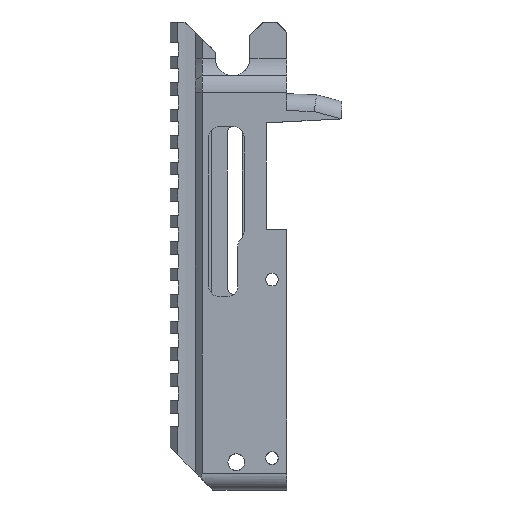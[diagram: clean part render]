
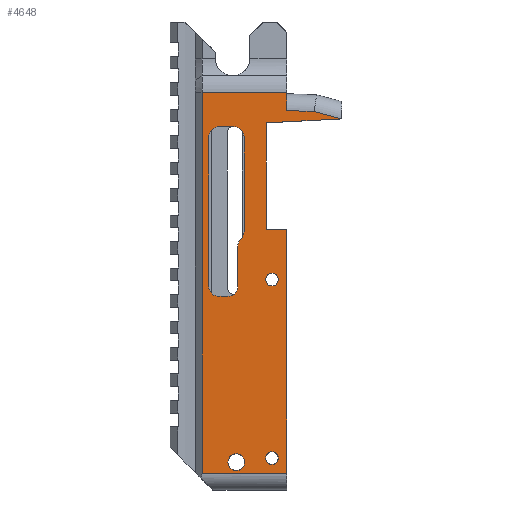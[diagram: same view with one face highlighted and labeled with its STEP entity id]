
A CAD part, left-side view. The second image highlights one B-rep face of the part: STEP entity #4648.
In plain terms, the highlighted planar face has unit normal (-1, 0, 0).
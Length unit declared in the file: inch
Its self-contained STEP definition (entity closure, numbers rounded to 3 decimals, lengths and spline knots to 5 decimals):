
#177=PLANE('',#7972);
#371=VECTOR('',#5113,1.);
#380=VECTOR('',#5125,1.);
#384=VECTOR('',#5140,1.);
#392=VECTOR('',#5170,1.);
#593=VECTOR('',#5457,1.);
#594=VECTOR('',#5460,1.);
#595=VECTOR('',#5463,1.);
#596=VECTOR('',#5466,1.);
#597=VECTOR('',#5469,1.);
#598=VECTOR('',#5472,1.);
#599=VECTOR('',#5473,1.);
#600=VECTOR('',#5474,1.);
#601=VECTOR('',#5475,1.);
#602=VECTOR('',#5476,1.);
#603=VECTOR('',#5477,1.);
#604=VECTOR('',#5478,1.);
#605=VECTOR('',#5479,1.);
#913=LINE('',#6662,#371);
#922=LINE('',#6680,#380);
#926=LINE('',#6695,#384);
#934=LINE('',#6792,#392);
#1135=LINE('',#7287,#593);
#1136=LINE('',#7291,#594);
#1137=LINE('',#7295,#595);
#1138=LINE('',#7299,#596);
#1139=LINE('',#7303,#597);
#1140=LINE('',#7307,#598);
#1141=LINE('',#7308,#599);
#1142=LINE('',#7311,#600);
#1143=LINE('',#7313,#601);
#1144=LINE('',#7314,#602);
#1145=LINE('',#7316,#603);
#1146=LINE('',#7318,#604);
#1147=LINE('',#7320,#605);
#1432=VERTEX_POINT('',#6313);
#1433=VERTEX_POINT('',#6314);
#1440=VERTEX_POINT('',#6354);
#1441=VERTEX_POINT('',#6355);
#1449=VERTEX_POINT('',#6407);
#1450=VERTEX_POINT('',#6408);
#1507=VERTEX_POINT('',#6661);
#1508=VERTEX_POINT('',#6663);
#1513=VERTEX_POINT('',#6679);
#1514=VERTEX_POINT('',#6681);
#1526=VERTEX_POINT('',#6791);
#1694=VERTEX_POINT('',#7285);
#1695=VERTEX_POINT('',#7286);
#1696=VERTEX_POINT('',#7288);
#1697=VERTEX_POINT('',#7290);
#1698=VERTEX_POINT('',#7292);
#1699=VERTEX_POINT('',#7294);
#1700=VERTEX_POINT('',#7296);
#1701=VERTEX_POINT('',#7298);
#1702=VERTEX_POINT('',#7300);
#1703=VERTEX_POINT('',#7302);
#1704=VERTEX_POINT('',#7304);
#1705=VERTEX_POINT('',#7306);
#1706=VERTEX_POINT('',#7309);
#1707=VERTEX_POINT('',#7310);
#1708=VERTEX_POINT('',#7312);
#1709=VERTEX_POINT('',#7315);
#1710=VERTEX_POINT('',#7317);
#1711=VERTEX_POINT('',#7319);
#1841=CIRCLE('',#7841,0.125);
#1844=CIRCLE('',#7846,0.09375);
#1848=CIRCLE('',#7852,0.09375);
#1867=CIRCLE('',#7891,0.09375);
#1869=CIRCLE('',#7893,0.09375);
#1871=CIRCLE('',#7895,0.125);
#1886=CIRCLE('',#7973,0.15);
#1887=CIRCLE('',#7974,0.15);
#1888=CIRCLE('',#7975,0.15);
#1889=CIRCLE('',#7976,0.15);
#1890=CIRCLE('',#7977,0.15);
#1891=CIRCLE('',#7978,0.15);
#2003=EDGE_CURVE('',#1432,#1433,#1841,.F.);
#2011=EDGE_CURVE('',#1440,#1441,#1844,.F.);
#2020=EDGE_CURVE('',#1449,#1450,#1848,.F.);
#2095=EDGE_CURVE('',#1507,#1508,#913,.T.);
#2104=EDGE_CURVE('',#1514,#1513,#922,.T.);
#2113=EDGE_CURVE('',#1508,#1513,#926,.F.);
#2115=EDGE_CURVE('',#1450,#1449,#1867,.F.);
#2119=EDGE_CURVE('',#1441,#1440,#1869,.F.);
#2121=EDGE_CURVE('',#1433,#1432,#1871,.F.);
#2132=EDGE_CURVE('',#1526,#1507,#934,.F.);
#2351=EDGE_CURVE('',#1694,#1695,#1886,.T.);
#2352=EDGE_CURVE('',#1696,#1694,#1135,.T.);
#2353=EDGE_CURVE('',#1697,#1696,#1887,.F.);
#2354=EDGE_CURVE('',#1698,#1697,#1136,.T.);
#2355=EDGE_CURVE('',#1699,#1698,#1888,.T.);
#2356=EDGE_CURVE('',#1700,#1699,#1137,.T.);
#2357=EDGE_CURVE('',#1701,#1700,#1889,.T.);
#2358=EDGE_CURVE('',#1702,#1701,#1138,.T.);
#2359=EDGE_CURVE('',#1703,#1702,#1890,.T.);
#2360=EDGE_CURVE('',#1704,#1703,#1139,.T.);
#2361=EDGE_CURVE('',#1705,#1704,#1891,.T.);
#2362=EDGE_CURVE('',#1695,#1705,#1140,.T.);
#2363=EDGE_CURVE('',#1706,#1707,#1141,.T.);
#2364=EDGE_CURVE('',#1707,#1708,#1142,.T.);
#2365=EDGE_CURVE('',#1708,#1514,#1143,.F.);
#2366=EDGE_CURVE('',#1526,#1709,#1144,.F.);
#2367=EDGE_CURVE('',#1709,#1710,#1145,.F.);
#2368=EDGE_CURVE('',#1710,#1711,#1146,.F.);
#2369=EDGE_CURVE('',#1711,#1706,#1147,.F.);
#3190=ORIENTED_EDGE('',*,*,#2351,.F.);
#3191=ORIENTED_EDGE('',*,*,#2352,.F.);
#3192=ORIENTED_EDGE('',*,*,#2353,.F.);
#3193=ORIENTED_EDGE('',*,*,#2354,.F.);
#3194=ORIENTED_EDGE('',*,*,#2355,.F.);
#3195=ORIENTED_EDGE('',*,*,#2356,.F.);
#3196=ORIENTED_EDGE('',*,*,#2357,.F.);
#3197=ORIENTED_EDGE('',*,*,#2358,.F.);
#3198=ORIENTED_EDGE('',*,*,#2359,.F.);
#3199=ORIENTED_EDGE('',*,*,#2360,.F.);
#3200=ORIENTED_EDGE('',*,*,#2361,.F.);
#3201=ORIENTED_EDGE('',*,*,#2362,.F.);
#3202=ORIENTED_EDGE('',*,*,#2363,.T.);
#3203=ORIENTED_EDGE('',*,*,#2364,.T.);
#3204=ORIENTED_EDGE('',*,*,#2365,.T.);
#3205=ORIENTED_EDGE('',*,*,#2104,.T.);
#3206=ORIENTED_EDGE('',*,*,#2113,.F.);
#3207=ORIENTED_EDGE('',*,*,#2095,.F.);
#3208=ORIENTED_EDGE('',*,*,#2132,.F.);
#3209=ORIENTED_EDGE('',*,*,#2366,.T.);
#3210=ORIENTED_EDGE('',*,*,#2367,.T.);
#3211=ORIENTED_EDGE('',*,*,#2368,.T.);
#3212=ORIENTED_EDGE('',*,*,#2369,.T.);
#3213=ORIENTED_EDGE('',*,*,#2003,.F.);
#3214=ORIENTED_EDGE('',*,*,#2121,.F.);
#3215=ORIENTED_EDGE('',*,*,#2011,.F.);
#3216=ORIENTED_EDGE('',*,*,#2119,.F.);
#3217=ORIENTED_EDGE('',*,*,#2020,.F.);
#3218=ORIENTED_EDGE('',*,*,#2115,.F.);
#4139=EDGE_LOOP('',(#3190,#3191,#3192,#3193,#3194,#3195,#3196,#3197,#3198,
#3199,#3200,#3201));
#4140=EDGE_LOOP('',(#3202,#3203,#3204,#3205,#3206,#3207,#3208,#3209,#3210,
#3211,#3212));
#4141=EDGE_LOOP('',(#3213,#3214));
#4142=EDGE_LOOP('',(#3215,#3216));
#4143=EDGE_LOOP('',(#3217,#3218));
#4398=FACE_BOUND('',#4139,.T.);
#4399=FACE_BOUND('',#4140,.T.);
#4400=FACE_BOUND('',#4141,.T.);
#4401=FACE_BOUND('',#4142,.T.);
#4402=FACE_BOUND('',#4143,.T.);
#4648=ADVANCED_FACE('',(#4398,#4399,#4400,#4401,#4402),#177,.T.);
#4981=DIRECTION('',(1.,0.,0.));
#4982=DIRECTION('',(0.,0.,-0.125));
#4995=DIRECTION('',(1.,0.,0.));
#4996=DIRECTION('',(0.,0.,-0.094));
#5011=DIRECTION('',(1.,0.,0.));
#5012=DIRECTION('',(0.,0.,-0.094));
#5113=DIRECTION('',(0.,0.,-1.));
#5125=DIRECTION('',(0.,0.,1.));
#5140=DIRECTION('',(0.,1.,0.));
#5143=DIRECTION('',(1.,0.,0.));
#5144=DIRECTION('',(0.,0.,-0.094));
#5147=DIRECTION('',(1.,0.,0.));
#5148=DIRECTION('',(0.,0.,-0.094));
#5151=DIRECTION('',(1.,0.,0.));
#5152=DIRECTION('',(0.,0.,-0.125));
#5170=DIRECTION('',(0.,-0.999,0.052));
#5454=DIRECTION('',(-1.,0.,0.));
#5455=DIRECTION('',(-1.,0.,0.));
#5456=DIRECTION('',(0.,0.,0.15));
#5457=DIRECTION('',(0.,-0.707,0.707));
#5458=DIRECTION('',(-1.,0.,0.));
#5459=DIRECTION('',(0.,0.,0.15));
#5460=DIRECTION('',(0.,0.,1.));
#5461=DIRECTION('',(-1.,0.,0.));
#5462=DIRECTION('',(0.,0.,0.15));
#5463=DIRECTION('',(0.,-1.,0.));
#5464=DIRECTION('',(-1.,0.,0.));
#5465=DIRECTION('',(0.,0.,0.15));
#5466=DIRECTION('',(0.,0.,-1.));
#5467=DIRECTION('',(-1.,0.,0.));
#5468=DIRECTION('',(0.,0.,0.15));
#5469=DIRECTION('',(0.,1.,0.));
#5470=DIRECTION('',(-1.,0.,0.));
#5471=DIRECTION('',(0.,0.,0.15));
#5472=DIRECTION('',(0.,0.,1.));
#5473=DIRECTION('',(0.,1.,0.));
#5474=DIRECTION('',(0.,0.,-1.));
#5475=DIRECTION('',(0.,1.,0.));
#5476=DIRECTION('',(0.,0.999,-0.052));
#5477=DIRECTION('',(0.,-0.966,-0.259));
#5478=DIRECTION('',(0.,-0.999,-0.039));
#5479=DIRECTION('',(0.,0.,-1.));
#6312=CARTESIAN_POINT('',(-0.625,0.75,-5.752));
#6313=CARTESIAN_POINT('',(-0.625,0.75,-5.877));
#6314=CARTESIAN_POINT('',(-0.625,0.75,-5.627));
#6353=CARTESIAN_POINT('',(-0.625,0.22,-3.035));
#6354=CARTESIAN_POINT('',(-0.625,0.22,-3.12875));
#6355=CARTESIAN_POINT('',(-0.625,0.22,-2.94125));
#6406=CARTESIAN_POINT('',(-0.625,0.22,-5.69));
#6407=CARTESIAN_POINT('',(-0.625,0.22,-5.78375));
#6408=CARTESIAN_POINT('',(-0.625,0.22,-5.59625));
#6661=CARTESIAN_POINT('',(-0.625,0.303,-0.70064));
#6662=CARTESIAN_POINT('',(-0.625,0.303,0.04972));
#6663=CARTESIAN_POINT('',(-0.625,0.303,-2.285));
#6679=CARTESIAN_POINT('',(-0.625,0.,-2.285));
#6680=CARTESIAN_POINT('',(-0.625,0.,0.0575));
#6681=CARTESIAN_POINT('',(-0.625,0.,-5.915));
#6695=CARTESIAN_POINT('',(-0.625,-0.41,-2.285));
#6698=CARTESIAN_POINT('',(-0.625,0.22,-5.69));
#6768=CARTESIAN_POINT('',(-0.625,0.22,-3.035));
#6770=CARTESIAN_POINT('',(-0.625,0.75,-5.752));
#6791=CARTESIAN_POINT('',(-0.625,0.00001,-0.68476));
#6792=CARTESIAN_POINT('',(-0.625,-0.24618,-0.67186));
#7283=CARTESIAN_POINT('',(-0.625,-0.82,0.8));
#7284=CARTESIAN_POINT('',(-0.625,0.785,-2.32037));
#7285=CARTESIAN_POINT('',(-0.625,0.67893,-2.42643));
#7286=CARTESIAN_POINT('',(-0.625,0.635,-2.32037));
#7287=CARTESIAN_POINT('',(-0.625,-0.50241,-1.24509));
#7288=CARTESIAN_POINT('',(-0.625,0.68607,-2.43357));
#7289=CARTESIAN_POINT('',(-0.625,0.58,-2.53963));
#7290=CARTESIAN_POINT('',(-0.625,0.73,-2.53963));
#7291=CARTESIAN_POINT('',(-0.625,0.73,-1.1675));
#7292=CARTESIAN_POINT('',(-0.625,0.73,-3.135));
#7293=CARTESIAN_POINT('',(-0.625,0.88,-3.135));
#7294=CARTESIAN_POINT('',(-0.625,0.88,-3.285));
#7295=CARTESIAN_POINT('',(-0.625,0.03,-3.285));
#7296=CARTESIAN_POINT('',(-0.625,1.01,-3.285));
#7297=CARTESIAN_POINT('',(-0.625,1.01,-3.135));
#7298=CARTESIAN_POINT('',(-0.625,1.16,-3.135));
#7299=CARTESIAN_POINT('',(-0.625,1.16,-0.05474));
#7300=CARTESIAN_POINT('',(-0.625,1.16,-0.90949));
#7301=CARTESIAN_POINT('',(-0.625,1.01,-0.90949));
#7302=CARTESIAN_POINT('',(-0.625,1.01,-0.75949));
#7303=CARTESIAN_POINT('',(-0.625,0.095,-0.75949));
#7304=CARTESIAN_POINT('',(-0.625,0.785,-0.75949));
#7305=CARTESIAN_POINT('',(-0.625,0.785,-0.90949));
#7306=CARTESIAN_POINT('',(-0.625,0.635,-0.90949));
#7307=CARTESIAN_POINT('',(-0.625,0.635,-0.76018));
#7308=CARTESIAN_POINT('',(-0.625,-0.82,-0.25));
#7309=CARTESIAN_POINT('',(-0.625,0.,-0.25));
#7310=CARTESIAN_POINT('',(-0.625,1.26,-0.25));
#7311=CARTESIAN_POINT('',(-0.625,1.26,0.8));
#7312=CARTESIAN_POINT('',(-0.625,1.26,-5.915));
#7313=CARTESIAN_POINT('',(-0.625,-0.82,-5.915));
#7314=CARTESIAN_POINT('',(-0.625,-0.44768,-0.66154));
#7315=CARTESIAN_POINT('',(-0.625,-0.81428,-0.64233));
#7316=CARTESIAN_POINT('',(-0.625,-0.45904,-0.54714));
#7317=CARTESIAN_POINT('',(-0.625,-0.40726,-0.53326));
#7318=CARTESIAN_POINT('',(-0.625,-0.76684,-0.54745));
#7319=CARTESIAN_POINT('',(-0.625,0.,-0.51719));
#7320=CARTESIAN_POINT('',(-0.625,0.,0.8));
#7841=AXIS2_PLACEMENT_3D('',#6312,#4981,#4982);
#7846=AXIS2_PLACEMENT_3D('',#6353,#4995,#4996);
#7852=AXIS2_PLACEMENT_3D('',#6406,#5011,#5012);
#7891=AXIS2_PLACEMENT_3D('',#6698,#5143,#5144);
#7893=AXIS2_PLACEMENT_3D('',#6768,#5147,#5148);
#7895=AXIS2_PLACEMENT_3D('',#6770,#5151,#5152);
#7972=AXIS2_PLACEMENT_3D('',#7283,#5454,$);
#7973=AXIS2_PLACEMENT_3D('',#7284,#5455,#5456);
#7974=AXIS2_PLACEMENT_3D('',#7289,#5458,#5459);
#7975=AXIS2_PLACEMENT_3D('',#7293,#5461,#5462);
#7976=AXIS2_PLACEMENT_3D('',#7297,#5464,#5465);
#7977=AXIS2_PLACEMENT_3D('',#7301,#5467,#5468);
#7978=AXIS2_PLACEMENT_3D('',#7305,#5470,#5471);
